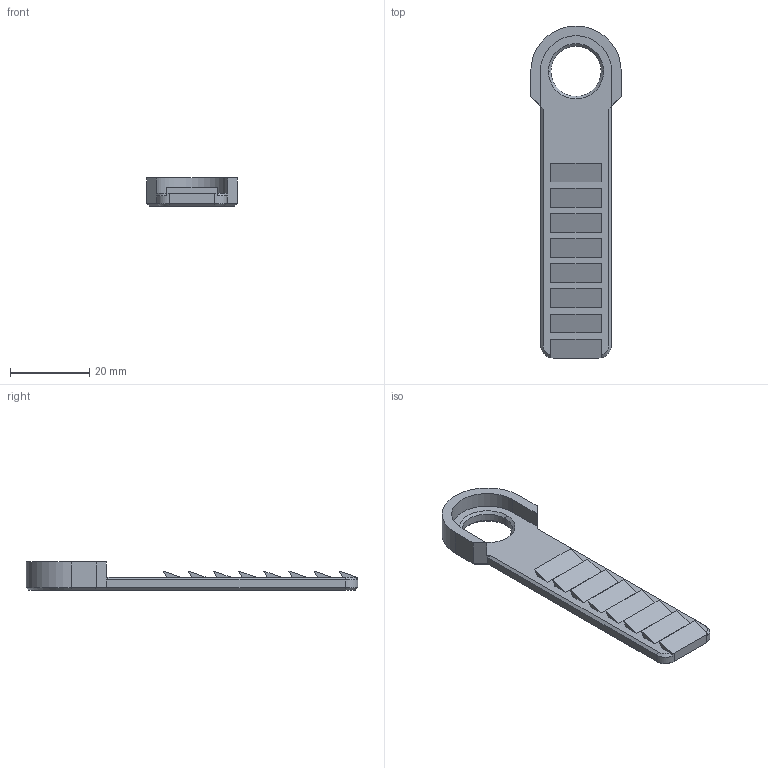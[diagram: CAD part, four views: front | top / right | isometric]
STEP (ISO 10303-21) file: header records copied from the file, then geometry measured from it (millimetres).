
FILE_DESCRIPTION (( 'STEP AP203' ), '1' );
FILE_NAME ('AF-GFP-AR15MP-PRT-004-STEP.STEP', '2020-08-23T10:14:12', ( '' ), ( '' ), 'SwSTEP 2.0', 'SolidWorks 2018', '' );
FILE_SCHEMA (( 'CONFIG_CONTROL_DESIGN' ));
Length unit declared in the file: inch
Products named in the file (1): AF-GFP-AR15MP-PRT-004-STEP
Bounding box: 22.86 x 83.82 x 7.09 mm (x, y, z)
Volume: 5091.6 mm3; surface area: 4322.7 mm2
Topology: 1 solids, 1 shells, 316 faces, 812 edges, 536 vertices
Faces by surface type: plane 238, bspline 63, cone 9, cylinder 6
Entity records: 13600 total; most frequent: CARTESIAN_POINT 6244, ORIENTED_EDGE 1624, DIRECTION 1211, EDGE_CURVE 812, VECTOR 661, LINE 661, VERTEX_POINT 536, EDGE_LOOP 356
